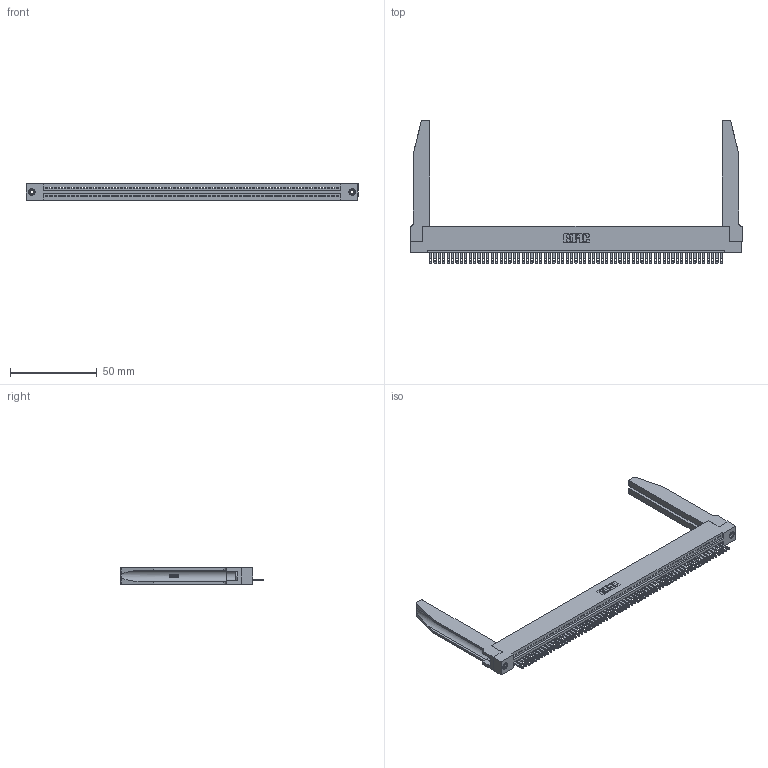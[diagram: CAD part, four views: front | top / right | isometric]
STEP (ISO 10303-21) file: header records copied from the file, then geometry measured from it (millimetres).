
FILE_DESCRIPTION (( 'STEP AP203' ), '1' );
FILE_NAME ('345-067-500-178.STEP', '2019-10-11T23:31:06', ( '' ), ( '' ), 'SwSTEP 2.0', 'SolidWorks 2016', '' );
FILE_SCHEMA (( 'CONFIG_CONTROL_DESIGN' ));
Length unit declared in the file: inch
Products named in the file (5): 345-220-078_345-220-078; 345 Part_Flush Mounting Lugs - 0.156 Dia-TH; 345-067-500-178; 345-250-001_345-250-001-102; 345-292-001_345-293-100
Assembly tree (72 placements, depth 2):
  345-067-500-178
    345 Part_Flush Mounting Lugs - 0.156 Dia-TH
    345-292-001_345-293-100  x67
    345-250-001_345-250-001-102  x2
    345-220-078_345-220-078  x2
Bounding box: 191.41 x 82.47 x 9.4 mm (x, y, z)
Volume: 26197.5 mm3; surface area: 31823.6 mm2
Topology: 72 solids, 72 shells, 3978 faces, 12205 edges, 8126 vertices
Faces by surface type: plane 2500, cylinder 1426, bspline 36, cone 12, torus 4
Entity records: 51730 total; most frequent: CARTESIAN_POINT 9856, ORIENTED_EDGE 8754, DIRECTION 7581, EDGE_CURVE 4377, LINE 3879, VECTOR 3879, VERTEX_POINT 2912, AXIS2_PLACEMENT_3D 1851
